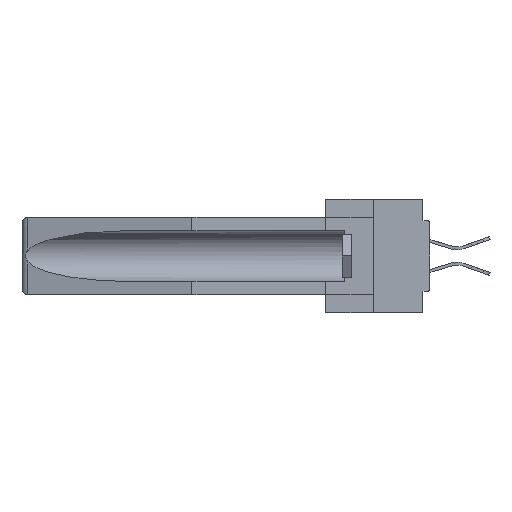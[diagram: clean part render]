
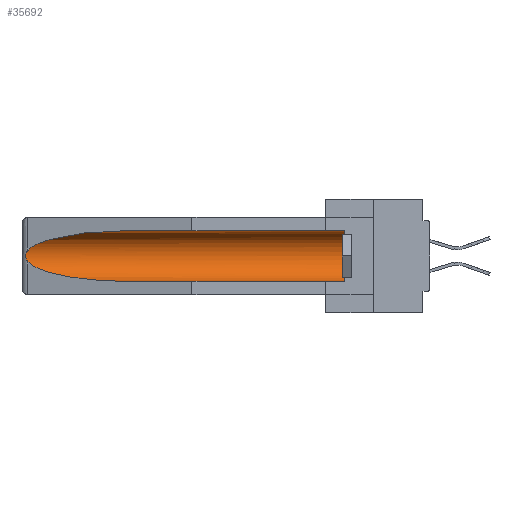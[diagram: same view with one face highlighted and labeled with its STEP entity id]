
A CAD part, left-side view. The second image highlights one B-rep face of the part: STEP entity #35692.
In plain terms, the highlighted cylindrical face has radius 2.857 mm (diameter 5.715 mm), a partial arc.
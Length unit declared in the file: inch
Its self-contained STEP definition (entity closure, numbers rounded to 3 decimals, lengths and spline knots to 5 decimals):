
#722 = CARTESIAN_POINT ( 'NONE',  ( 0.155, 1.07973, -0.059 ) ) ;
#744 = VERTEX_POINT ( 'NONE', #722 ) ;
#966 = CARTESIAN_POINT ( 'NONE',  ( 0.26597, 1.5296, -0.19026 ) ) ;
#1226 = ORIENTED_EDGE ( 'NONE', *, *, #2266, .T. ) ;
#2266 = EDGE_CURVE ( 'NONE', #3513, #11283, #11950, .T. ) ;
#3287 = CARTESIAN_POINT ( 'NONE',  ( 0.26537, 1.52718, -0.14972 ) ) ;
#3415 = EDGE_CURVE ( 'NONE', #21172, #5323, #37578, .T. ) ;
#3423 = VECTOR ( 'NONE', #34682, 39.37008 ) ;
#3513 = VERTEX_POINT ( 'NONE', #32501 ) ;
#3870 = FACE_OUTER_BOUND ( 'NONE', #16819, .T. ) ;
#4921 = EDGE_CURVE ( 'NONE', #744, #11825, #30721, .T. ) ;
#5323 = VERTEX_POINT ( 'NONE', #21925 ) ;
#5397 = CARTESIAN_POINT ( 'NONE',  ( 0.155, 1.07973, -0.284 ) ) ;
#5851 = CARTESIAN_POINT ( 'NONE',  ( 0.155, -0.30754, -0.284 ) ) ;
#6122 = DIRECTION ( 'NONE',  ( 0., 1., 0. ) ) ;
#7830 = CARTESIAN_POINT ( 'NONE',  ( 0.155, 1.07973, -0.284 ) ) ;
#8081 = DIRECTION ( 'NONE',  ( 0., 1., 0. ) ) ;
#9182 = CARTESIAN_POINT ( 'NONE',  ( 0.26597, 1.52961, -0.15275 ) ) ;
#9210 = ORIENTED_EDGE ( 'NONE', *, *, #25202, .F. ) ;
#10169 = CARTESIAN_POINT ( 'NONE',  ( 0.155, 1.07973, -0.059 ) ) ;
#10316 = B_SPLINE_CURVE_WITH_KNOTS ( 'NONE', 3,
 ( #3287, #9182, #17731, #35554, #11628, #32728, #18396, #23896, #966, #21090 ),
 .UNSPECIFIED., .F., .F.,
 ( 4, 2, 2, 2, 4 ),
 ( 0., 0.00029, 0.00058, 0.00087, 0.00117 ),
 .UNSPECIFIED. ) ;
#11283 = VERTEX_POINT ( 'NONE', #5397 ) ;
#11424 = CARTESIAN_POINT ( 'NONE',  ( 0.155, -0.30754, -0.059 ) ) ;
#11628 = CARTESIAN_POINT ( 'NONE',  ( 0.2675, 1.53308, -0.16763 ) ) ;
#11825 = VERTEX_POINT ( 'NONE', #33237 ) ;
#11880 = DIRECTION ( 'NONE',  ( 0., 0., 1. ) ) ;
#11950 =( BOUNDED_CURVE ( )  B_SPLINE_CURVE ( 3, ( #36421, #27822, #30771, #7830 ),
 .UNSPECIFIED., .F., .F. ) 
 B_SPLINE_CURVE_WITH_KNOTS ( ( 4, 4 ),
 ( 0.1948, 1.5708 ),
 .UNSPECIFIED. ) 
 CURVE ( )  GEOMETRIC_REPRESENTATION_ITEM ( )  RATIONAL_B_SPLINE_CURVE ( ( 1., 0.848, 0.848, 1. ) ) 
 REPRESENTATION_ITEM ( '' )  );
#13375 = CARTESIAN_POINT ( 'NONE',  ( 0.21114, 1.30732, -0.059 ) ) ;
#14495 = AXIS2_PLACEMENT_3D ( 'NONE', #17220, #17094, #11880 ) ;
#16819 = EDGE_LOOP ( 'NONE', ( #35309, #22141, #1226, #9210, #17652, #17226 ) ) ;
#17094 = DIRECTION ( 'NONE',  ( 0., -1., 0. ) ) ;
#17220 = CARTESIAN_POINT ( 'NONE',  ( 0.155, 0.126, -0.1715 ) ) ;
#17226 = ORIENTED_EDGE ( 'NONE', *, *, #25152, .T. ) ;
#17652 = ORIENTED_EDGE ( 'NONE', *, *, #3415, .T. ) ;
#17731 = CARTESIAN_POINT ( 'NONE',  ( 0.26654, 1.53092, -0.15636 ) ) ;
#18396 = CARTESIAN_POINT ( 'NONE',  ( 0.2673, 1.53269, -0.17917 ) ) ;
#18428 = CARTESIAN_POINT ( 'NONE',  ( 0.155, 0.126, -0.284 ) ) ;
#19224 = CARTESIAN_POINT ( 'NONE',  ( 0.25451, 1.48313, -0.09465 ) ) ;
#21090 = CARTESIAN_POINT ( 'NONE',  ( 0.26537, 1.52718, -0.19328 ) ) ;
#21172 = VERTEX_POINT ( 'NONE', #18428 ) ;
#21925 = CARTESIAN_POINT ( 'NONE',  ( 0.155, 0.126, -0.059 ) ) ;
#22141 = ORIENTED_EDGE ( 'NONE', *, *, #30063, .T. ) ;
#22182 = CARTESIAN_POINT ( 'NONE',  ( 0.26537, 1.52718, -0.14972 ) ) ;
#23896 = CARTESIAN_POINT ( 'NONE',  ( 0.26655, 1.53094, -0.18657 ) ) ;
#25152 = EDGE_CURVE ( 'NONE', #5323, #744, #34101, .T. ) ;
#25202 = EDGE_CURVE ( 'NONE', #21172, #11283, #26779, .T. ) ;
#26298 = VECTOR ( 'NONE', #8081, 39.37008 ) ;
#26302 = CYLINDRICAL_SURFACE ( 'NONE', #29444, 0.1125 ) ;
#26365 = CARTESIAN_POINT ( 'NONE',  ( 0.155, -0.30754, -0.1715 ) ) ;
#26779 = LINE ( 'NONE', #5851, #3423 ) ;
#27822 = CARTESIAN_POINT ( 'NONE',  ( 0.25451, 1.48313, -0.24835 ) ) ;
#29444 = AXIS2_PLACEMENT_3D ( 'NONE', #26365, #6122, #29957 ) ;
#29957 = DIRECTION ( 'NONE',  ( 0., 0., 1. ) ) ;
#30063 = EDGE_CURVE ( 'NONE', #11825, #3513, #10316, .T. ) ;
#30721 =( BOUNDED_CURVE ( )  B_SPLINE_CURVE ( 3, ( #10169, #13375, #19224, #22182 ),
 .UNSPECIFIED., .F., .F. ) 
 B_SPLINE_CURVE_WITH_KNOTS ( ( 4, 4 ),
 ( 4.71239, 6.08839 ),
 .UNSPECIFIED. ) 
 CURVE ( )  GEOMETRIC_REPRESENTATION_ITEM ( )  RATIONAL_B_SPLINE_CURVE ( ( 1., 0.848, 0.848, 1. ) ) 
 REPRESENTATION_ITEM ( '' )  );
#30771 = CARTESIAN_POINT ( 'NONE',  ( 0.21114, 1.30732, -0.284 ) ) ;
#32501 = CARTESIAN_POINT ( 'NONE',  ( 0.26537, 1.52718, -0.19328 ) ) ;
#32728 = CARTESIAN_POINT ( 'NONE',  ( 0.2675, 1.53308, -0.17534 ) ) ;
#33237 = CARTESIAN_POINT ( 'NONE',  ( 0.26537, 1.52718, -0.14972 ) ) ;
#34101 = LINE ( 'NONE', #11424, #26298 ) ;
#34682 = DIRECTION ( 'NONE',  ( 0., 1., 0. ) ) ;
#35309 = ORIENTED_EDGE ( 'NONE', *, *, #4921, .T. ) ;
#35554 = CARTESIAN_POINT ( 'NONE',  ( 0.2673, 1.5327, -0.16383 ) ) ;
#35692 = ADVANCED_FACE ( 'NONE', ( #3870 ), #26302, .F. ) ;
#36421 = CARTESIAN_POINT ( 'NONE',  ( 0.26537, 1.52718, -0.19328 ) ) ;
#37578 = CIRCLE ( 'NONE', #14495, 0.1125 ) ;
